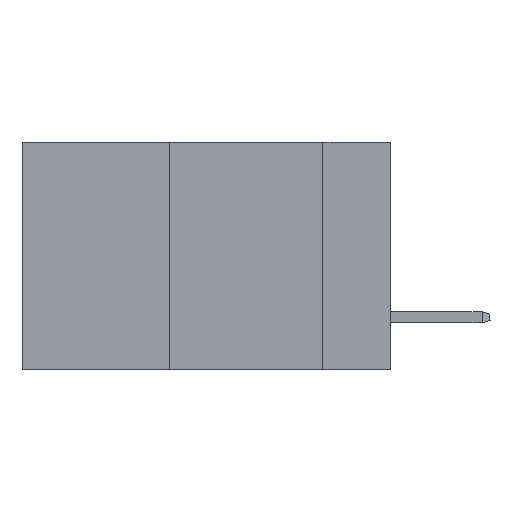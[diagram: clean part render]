
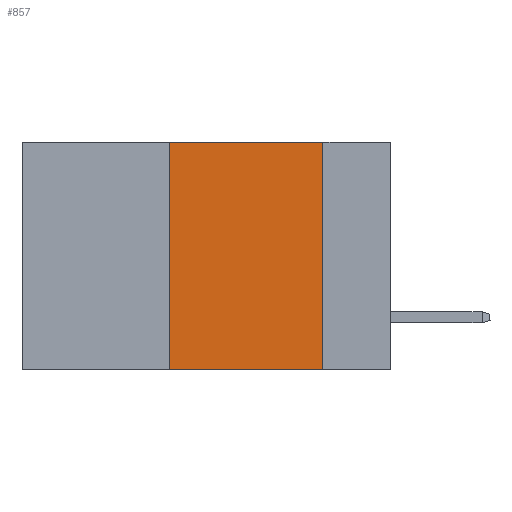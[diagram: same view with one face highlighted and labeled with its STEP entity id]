
A CAD part, left-side view. The second image highlights one B-rep face of the part: STEP entity #857.
In plain terms, the highlighted planar face has unit normal (-1, 0, 0).
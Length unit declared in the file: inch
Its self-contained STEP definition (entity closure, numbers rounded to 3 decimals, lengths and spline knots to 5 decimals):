
#857 = ADVANCED_FACE ( 'NONE', ( #29158 ), #14172, .F. ) ;
#1731 = CARTESIAN_POINT ( 'NONE',  ( 0., 0.11, -0.37 ) ) ;
#2823 = AXIS2_PLACEMENT_3D ( 'NONE', #16697, #24444, #29321 ) ;
#3002 = ORIENTED_EDGE ( 'NONE', *, *, #11644, .T. ) ;
#3110 = VERTEX_POINT ( 'NONE', #13000 ) ;
#3377 = CARTESIAN_POINT ( 'NONE',  ( 0., 0.11, 0. ) ) ;
#5784 = DIRECTION ( 'NONE',  ( 0., 0., -1. ) ) ;
#8252 = CARTESIAN_POINT ( 'NONE',  ( 0., 0.6, 0. ) ) ;
#11644 = EDGE_CURVE ( 'NONE', #22050, #23389, #11869, .T. ) ;
#11656 = EDGE_CURVE ( 'NONE', #22050, #29332, #22384, .T. ) ;
#11869 = LINE ( 'NONE', #26263, #13378 ) ;
#12686 = EDGE_CURVE ( 'NONE', #3110, #23389, #21889, .T. ) ;
#13000 = CARTESIAN_POINT ( 'NONE',  ( 0., 0.11, 0. ) ) ;
#13378 = VECTOR ( 'NONE', #23999, 39.37008 ) ;
#14172 = PLANE ( 'NONE',  #2823 ) ;
#16136 = CARTESIAN_POINT ( 'NONE',  ( 0., 0.36, -0.37 ) ) ;
#16697 = CARTESIAN_POINT ( 'NONE',  ( 0., 0.6, 0. ) ) ;
#16757 = CARTESIAN_POINT ( 'NONE',  ( 0., 0.36, 0. ) ) ;
#16795 = EDGE_CURVE ( 'NONE', #29332, #3110, #17288, .T. ) ;
#17288 = LINE ( 'NONE', #8252, #22191 ) ;
#17475 = VECTOR ( 'NONE', #23863, 39.37008 ) ;
#21889 = LINE ( 'NONE', #3377, #30617 ) ;
#22050 = VERTEX_POINT ( 'NONE', #16136 ) ;
#22191 = VECTOR ( 'NONE', #25079, 39.37008 ) ;
#22384 = LINE ( 'NONE', #16757, #17475 ) ;
#23389 = VERTEX_POINT ( 'NONE', #1731 ) ;
#23863 = DIRECTION ( 'NONE',  ( 0., 0., 1. ) ) ;
#23943 = ORIENTED_EDGE ( 'NONE', *, *, #11656, .F. ) ;
#23999 = DIRECTION ( 'NONE',  ( 0., -1., 0. ) ) ;
#24444 = DIRECTION ( 'NONE',  ( 1., 0., 0. ) ) ;
#25079 = DIRECTION ( 'NONE',  ( 0., -1., 0. ) ) ;
#25684 = ORIENTED_EDGE ( 'NONE', *, *, #16795, .F. ) ;
#26263 = CARTESIAN_POINT ( 'NONE',  ( 0., 0.6, -0.37 ) ) ;
#27652 = ORIENTED_EDGE ( 'NONE', *, *, #12686, .F. ) ;
#28178 = EDGE_LOOP ( 'NONE', ( #27652, #25684, #23943, #3002 ) ) ;
#29158 = FACE_OUTER_BOUND ( 'NONE', #28178, .T. ) ;
#29321 = DIRECTION ( 'NONE',  ( 0., 0., -1. ) ) ;
#29332 = VERTEX_POINT ( 'NONE', #31156 ) ;
#30617 = VECTOR ( 'NONE', #5784, 39.37008 ) ;
#31156 = CARTESIAN_POINT ( 'NONE',  ( 0., 0.36, 0. ) ) ;
